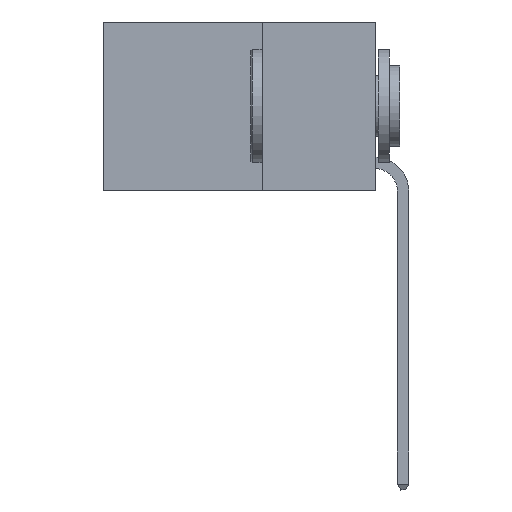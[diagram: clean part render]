
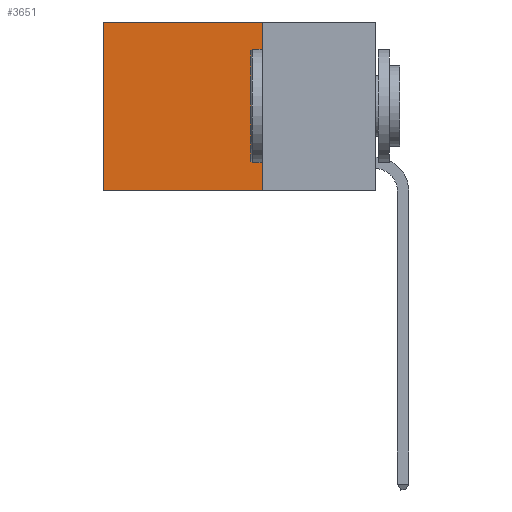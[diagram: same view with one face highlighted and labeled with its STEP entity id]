
A CAD part, left-side view. The second image highlights one B-rep face of the part: STEP entity #3651.
In plain terms, the highlighted planar face has unit normal (-1, 0, 0).
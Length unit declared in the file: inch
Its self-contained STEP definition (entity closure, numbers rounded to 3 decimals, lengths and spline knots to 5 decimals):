
#19 = CARTESIAN_POINT ( 'NONE',  ( 0.2625, 0.25, 0. ) ) ;
#39 = DIRECTION ( 'NONE',  ( 0., 1., 0. ) ) ;
#233 = ORIENTED_EDGE ( 'NONE', *, *, #1248, .F. ) ;
#241 = VERTEX_POINT ( 'NONE', #5079 ) ;
#991 = CARTESIAN_POINT ( 'NONE',  ( 0.2625, 0.6, -0.37 ) ) ;
#1248 = EDGE_CURVE ( 'NONE', #241, #12629, #7747, .T. ) ;
#1370 = ORIENTED_EDGE ( 'NONE', *, *, #11669, .T. ) ;
#1914 = LINE ( 'NONE', #8986, #2275 ) ;
#2275 = VECTOR ( 'NONE', #3322, 39.37008 ) ;
#3322 = DIRECTION ( 'NONE',  ( 0., 0., -1. ) ) ;
#3365 = ORIENTED_EDGE ( 'NONE', *, *, #9216, .T. ) ;
#3651 = ADVANCED_FACE ( 'NONE', ( #14539 ), #12292, .F. ) ;
#3787 = VECTOR ( 'NONE', #39, 39.37008 ) ;
#4036 = LINE ( 'NONE', #7526, #9372 ) ;
#4322 = VERTEX_POINT ( 'NONE', #19 ) ;
#5079 = CARTESIAN_POINT ( 'NONE',  ( 0.2625, 0.25, -0.37 ) ) ;
#5484 = AXIS2_PLACEMENT_3D ( 'NONE', #12390, #12205, #12055 ) ;
#5908 = ORIENTED_EDGE ( 'NONE', *, *, #14353, .F. ) ;
#6337 = DIRECTION ( 'NONE',  ( 0., 0., -1. ) ) ;
#7526 = CARTESIAN_POINT ( 'NONE',  ( 0.2625, 0.6, 0. ) ) ;
#7661 = VECTOR ( 'NONE', #7713, 39.37008 ) ;
#7713 = DIRECTION ( 'NONE',  ( 0., 1., 0. ) ) ;
#7747 = LINE ( 'NONE', #9269, #7661 ) ;
#8986 = CARTESIAN_POINT ( 'NONE',  ( 0.2625, 0.25, 0. ) ) ;
#9216 = EDGE_CURVE ( 'NONE', #11698, #12629, #4036, .T. ) ;
#9269 = CARTESIAN_POINT ( 'NONE',  ( 0.2625, 0.25, -0.37 ) ) ;
#9372 = VECTOR ( 'NONE', #6337, 39.37008 ) ;
#11669 = EDGE_CURVE ( 'NONE', #4322, #11698, #12773, .T. ) ;
#11698 = VERTEX_POINT ( 'NONE', #13692 ) ;
#12055 = DIRECTION ( 'NONE',  ( 0., 0., -1. ) ) ;
#12205 = DIRECTION ( 'NONE',  ( 1., 0., 0. ) ) ;
#12292 = PLANE ( 'NONE',  #5484 ) ;
#12390 = CARTESIAN_POINT ( 'NONE',  ( 0.2625, 0.25, 0. ) ) ;
#12629 = VERTEX_POINT ( 'NONE', #991 ) ;
#12773 = LINE ( 'NONE', #13647, #3787 ) ;
#12884 = EDGE_LOOP ( 'NONE', ( #3365, #233, #5908, #1370 ) ) ;
#13647 = CARTESIAN_POINT ( 'NONE',  ( 0.2625, 0.25, 0. ) ) ;
#13692 = CARTESIAN_POINT ( 'NONE',  ( 0.2625, 0.6, 0. ) ) ;
#14353 = EDGE_CURVE ( 'NONE', #4322, #241, #1914, .T. ) ;
#14539 = FACE_OUTER_BOUND ( 'NONE', #12884, .T. ) ;
